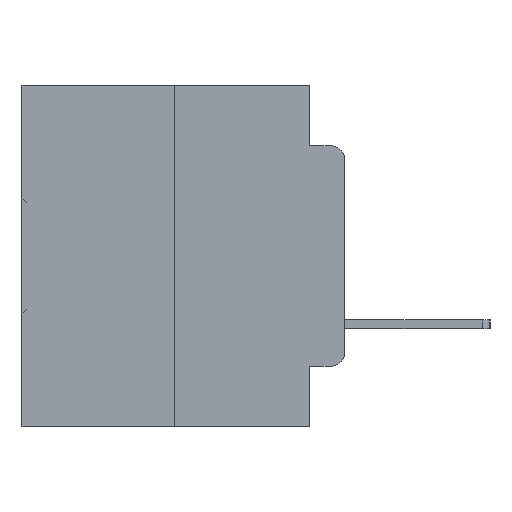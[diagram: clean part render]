
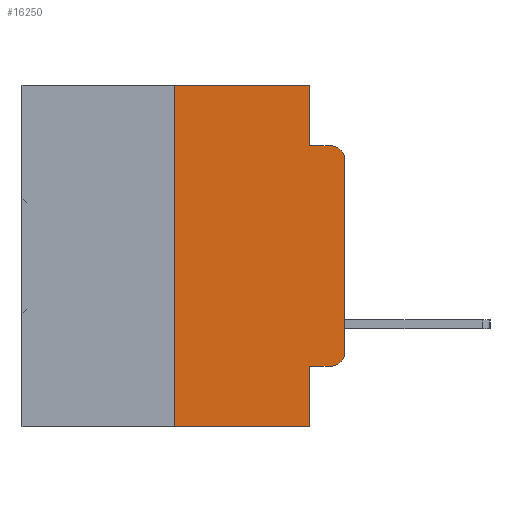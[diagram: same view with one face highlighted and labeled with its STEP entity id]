
A CAD part, left-side view. The second image highlights one B-rep face of the part: STEP entity #16250.
In plain terms, the highlighted planar face has unit normal (-1, 0, 0).
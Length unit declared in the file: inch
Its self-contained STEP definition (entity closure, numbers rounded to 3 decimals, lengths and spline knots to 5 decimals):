
#598 = CARTESIAN_POINT ( 'NONE',  ( 0., 0.473, 0. ) ) ;
#695 = LINE ( 'NONE', #22440, #22216 ) ;
#983 = EDGE_CURVE ( 'NONE', #11828, #31498, #5425, .T. ) ;
#1275 = VECTOR ( 'NONE', #21700, 39.37008 ) ;
#1431 = EDGE_CURVE ( 'NONE', #3799, #31176, #18677, .T. ) ;
#1642 = ORIENTED_EDGE ( 'NONE', *, *, #27362, .T. ) ;
#1711 = VECTOR ( 'NONE', #30027, 39.37008 ) ;
#1951 = CARTESIAN_POINT ( 'NONE',  ( 0., 0.25, -0.5 ) ) ;
#2049 = ORIENTED_EDGE ( 'NONE', *, *, #1431, .T. ) ;
#2085 = LINE ( 'NONE', #8518, #8713 ) ;
#3244 = ORIENTED_EDGE ( 'NONE', *, *, #4169, .T. ) ;
#3382 = CARTESIAN_POINT ( 'NONE',  ( 0., 0., 0. ) ) ;
#3619 = ORIENTED_EDGE ( 'NONE', *, *, #983, .F. ) ;
#3799 = VERTEX_POINT ( 'NONE', #29458 ) ;
#3977 = CARTESIAN_POINT ( 'NONE',  ( 0., 0.02, -0.1085 ) ) ;
#4169 = EDGE_CURVE ( 'NONE', #20974, #3799, #30325, .T. ) ;
#5176 = ORIENTED_EDGE ( 'NONE', *, *, #10669, .F. ) ;
#5425 = LINE ( 'NONE', #20220, #30876 ) ;
#6270 = VERTEX_POINT ( 'NONE', #15046 ) ;
#6479 = DIRECTION ( 'NONE',  ( 0., 0., -1. ) ) ;
#7996 = DIRECTION ( 'NONE',  ( 0., -1., 0. ) ) ;
#8518 = CARTESIAN_POINT ( 'NONE',  ( 0., 0.473, -0.5 ) ) ;
#8713 = VECTOR ( 'NONE', #13441, 39.37008 ) ;
#8784 = DIRECTION ( 'NONE',  ( 0., 0., 1. ) ) ;
#9126 = EDGE_LOOP ( 'NONE', ( #2049, #16121, #3619, #16530, #16913, #5176, #18452, #14980, #1642, #3244 ) ) ;
#10669 = EDGE_CURVE ( 'NONE', #29759, #13110, #21336, .T. ) ;
#10822 = CARTESIAN_POINT ( 'NONE',  ( 0., 0.051, -0.0885 ) ) ;
#11083 = VECTOR ( 'NONE', #23453, 39.37008 ) ;
#11626 = VERTEX_POINT ( 'NONE', #17264 ) ;
#11720 = CARTESIAN_POINT ( 'NONE',  ( 0., 0.02, -0.4115 ) ) ;
#11727 = EDGE_CURVE ( 'NONE', #11626, #11828, #21649, .T. ) ;
#11828 = VERTEX_POINT ( 'NONE', #10822 ) ;
#11854 = CARTESIAN_POINT ( 'NONE',  ( 0., 0.02, -0.3915 ) ) ;
#11868 = LINE ( 'NONE', #30633, #11083 ) ;
#12794 = EDGE_CURVE ( 'NONE', #29759, #24341, #2085, .T. ) ;
#12837 = VECTOR ( 'NONE', #15834, 39.37008 ) ;
#13110 = VERTEX_POINT ( 'NONE', #24557 ) ;
#13441 = DIRECTION ( 'NONE',  ( 0., -1., 0. ) ) ;
#13715 = AXIS2_PLACEMENT_3D ( 'NONE', #11854, #29024, #14377 ) ;
#14377 = DIRECTION ( 'NONE',  ( 0., 0., -1. ) ) ;
#14637 = LINE ( 'NONE', #21591, #1275 ) ;
#14980 = ORIENTED_EDGE ( 'NONE', *, *, #19639, .F. ) ;
#15046 = CARTESIAN_POINT ( 'NONE',  ( 0., 0.051, -0.4115 ) ) ;
#15408 = CARTESIAN_POINT ( 'NONE',  ( 0., 0.051, 0. ) ) ;
#15748 = DIRECTION ( 'NONE',  ( 0., 0., -1. ) ) ;
#15834 = DIRECTION ( 'NONE',  ( 0., 0., 1. ) ) ;
#16121 = ORIENTED_EDGE ( 'NONE', *, *, #25981, .T. ) ;
#16250 = ADVANCED_FACE ( 'NONE', ( #28911 ), #23082, .F. ) ;
#16530 = ORIENTED_EDGE ( 'NONE', *, *, #11727, .F. ) ;
#16729 = CARTESIAN_POINT ( 'NONE',  ( 0., 0.02, -0.0885 ) ) ;
#16913 = ORIENTED_EDGE ( 'NONE', *, *, #19307, .F. ) ;
#17264 = CARTESIAN_POINT ( 'NONE',  ( 0., 0.051, 0. ) ) ;
#17404 = CARTESIAN_POINT ( 'NONE',  ( 0., 0.051, -0.5 ) ) ;
#18452 = ORIENTED_EDGE ( 'NONE', *, *, #12794, .T. ) ;
#18677 = LINE ( 'NONE', #3382, #12837 ) ;
#19307 = EDGE_CURVE ( 'NONE', #13110, #11626, #14637, .T. ) ;
#19639 = EDGE_CURVE ( 'NONE', #6270, #24341, #11868, .T. ) ;
#20220 = CARTESIAN_POINT ( 'NONE',  ( 0., 0.051, -0.0885 ) ) ;
#20542 = VECTOR ( 'NONE', #8784, 39.37008 ) ;
#20974 = VERTEX_POINT ( 'NONE', #11720 ) ;
#21336 = LINE ( 'NONE', #26091, #20542 ) ;
#21427 = DIRECTION ( 'NONE',  ( -1., 0., 0. ) ) ;
#21591 = CARTESIAN_POINT ( 'NONE',  ( 0., 0.473, 0. ) ) ;
#21649 = LINE ( 'NONE', #15408, #1711 ) ;
#21700 = DIRECTION ( 'NONE',  ( 0., -1., 0. ) ) ;
#22216 = VECTOR ( 'NONE', #32045, 39.37008 ) ;
#22440 = CARTESIAN_POINT ( 'NONE',  ( 0., 0.051, -0.4115 ) ) ;
#23082 = PLANE ( 'NONE',  #29667 ) ;
#23453 = DIRECTION ( 'NONE',  ( 0., 0., -1. ) ) ;
#24341 = VERTEX_POINT ( 'NONE', #17404 ) ;
#24557 = CARTESIAN_POINT ( 'NONE',  ( 0., 0.25, 0. ) ) ;
#25981 = EDGE_CURVE ( 'NONE', #31176, #31498, #27936, .T. ) ;
#26091 = CARTESIAN_POINT ( 'NONE',  ( 0., 0.25, 0. ) ) ;
#26445 = AXIS2_PLACEMENT_3D ( 'NONE', #3977, #21427, #6479 ) ;
#27362 = EDGE_CURVE ( 'NONE', #6270, #20974, #695, .T. ) ;
#27936 = CIRCLE ( 'NONE', #26445, 0.02 ) ;
#28911 = FACE_OUTER_BOUND ( 'NONE', #9126, .T. ) ;
#29024 = DIRECTION ( 'NONE',  ( -1., 0., 0. ) ) ;
#29458 = CARTESIAN_POINT ( 'NONE',  ( 0., 0., -0.3915 ) ) ;
#29630 = CARTESIAN_POINT ( 'NONE',  ( 0., 0., -0.1085 ) ) ;
#29667 = AXIS2_PLACEMENT_3D ( 'NONE', #598, #30365, #15748 ) ;
#29759 = VERTEX_POINT ( 'NONE', #1951 ) ;
#30027 = DIRECTION ( 'NONE',  ( 0., 0., -1. ) ) ;
#30325 = CIRCLE ( 'NONE', #13715, 0.02 ) ;
#30365 = DIRECTION ( 'NONE',  ( 1., 0., 0. ) ) ;
#30633 = CARTESIAN_POINT ( 'NONE',  ( 0., 0.051, 0. ) ) ;
#30876 = VECTOR ( 'NONE', #7996, 39.37008 ) ;
#31176 = VERTEX_POINT ( 'NONE', #29630 ) ;
#31498 = VERTEX_POINT ( 'NONE', #16729 ) ;
#32045 = DIRECTION ( 'NONE',  ( 0., -1., 0. ) ) ;
